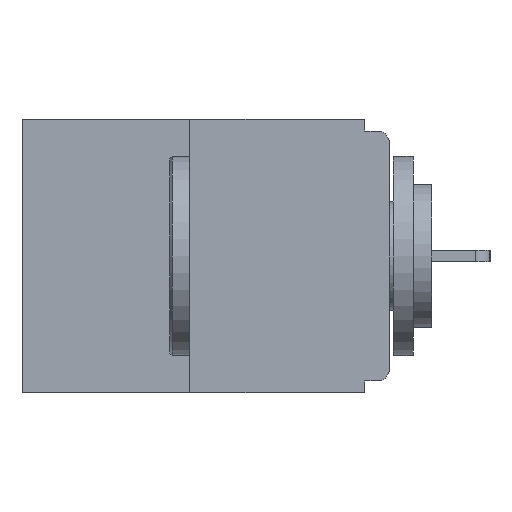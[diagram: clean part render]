
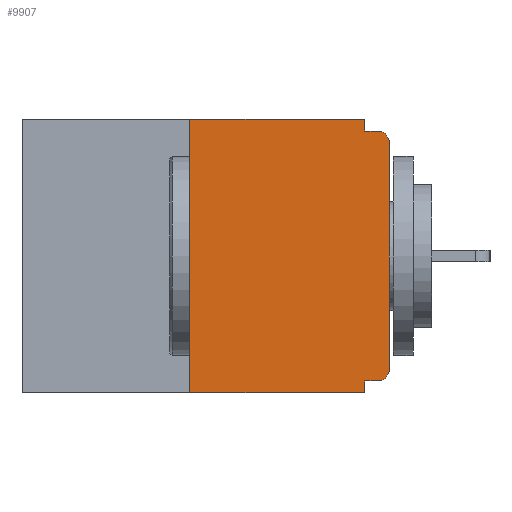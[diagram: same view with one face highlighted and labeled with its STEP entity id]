
A CAD part, left-side view. The second image highlights one B-rep face of the part: STEP entity #9907.
In plain terms, the highlighted planar face has unit normal (-1, 0, 0).
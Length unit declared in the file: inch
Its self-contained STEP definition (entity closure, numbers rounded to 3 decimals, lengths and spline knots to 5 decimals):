
#14 = CIRCLE ( 'NONE', #12090, 0.015 ) ;
#15 = VECTOR ( 'NONE', #4127, 39.37008 ) ;
#168 = VERTEX_POINT ( 'NONE', #7104 ) ;
#315 = CARTESIAN_POINT ( 'NONE',  ( 0., 0.031, -0.343 ) ) ;
#317 = VECTOR ( 'NONE', #24009, 39.37008 ) ;
#413 = CARTESIAN_POINT ( 'NONE',  ( 0., 0., -0.015 ) ) ;
#1266 = VERTEX_POINT ( 'NONE', #2147 ) ;
#1448 = ORIENTED_EDGE ( 'NONE', *, *, #12401, .F. ) ;
#2147 = CARTESIAN_POINT ( 'NONE',  ( 0., 0.031, -0.015 ) ) ;
#2425 = DIRECTION ( 'NONE',  ( 0., 0., -1. ) ) ;
#2603 = DIRECTION ( 'NONE',  ( 0., -1., 0. ) ) ;
#2755 = ORIENTED_EDGE ( 'NONE', *, *, #16962, .F. ) ;
#2942 = VERTEX_POINT ( 'NONE', #4803 ) ;
#3074 = EDGE_CURVE ( 'NONE', #17385, #5386, #14, .T. ) ;
#3148 = LINE ( 'NONE', #9006, #18382 ) ;
#3229 = AXIS2_PLACEMENT_3D ( 'NONE', #9556, #23301, #11506 ) ;
#4127 = DIRECTION ( 'NONE',  ( 0., -1., 0. ) ) ;
#4778 = VECTOR ( 'NONE', #25090, 39.37008 ) ;
#4803 = CARTESIAN_POINT ( 'NONE',  ( 0., 0.031, -0.328 ) ) ;
#5386 = VERTEX_POINT ( 'NONE', #9613 ) ;
#5591 = EDGE_LOOP ( 'NONE', ( #2755, #8173, #11188, #17680, #1448, #23832, #8790, #19927, #10609, #21147 ) ) ;
#5825 = EDGE_CURVE ( 'NONE', #1266, #168, #15173, .T. ) ;
#6660 = CARTESIAN_POINT ( 'NONE',  ( 0., 0.25, 0. ) ) ;
#7104 = CARTESIAN_POINT ( 'NONE',  ( 0., 0.015, -0.015 ) ) ;
#7207 = LINE ( 'NONE', #8399, #22310 ) ;
#8173 = ORIENTED_EDGE ( 'NONE', *, *, #24407, .F. ) ;
#8399 = CARTESIAN_POINT ( 'NONE',  ( 0., 0.46, -0.343 ) ) ;
#8790 = ORIENTED_EDGE ( 'NONE', *, *, #19071, .T. ) ;
#8882 = VERTEX_POINT ( 'NONE', #12332 ) ;
#9006 = CARTESIAN_POINT ( 'NONE',  ( 0., 0., 0. ) ) ;
#9134 = VECTOR ( 'NONE', #16734, 39.37008 ) ;
#9327 = CARTESIAN_POINT ( 'NONE',  ( 0., 0.015, -0.328 ) ) ;
#9354 = VERTEX_POINT ( 'NONE', #23588 ) ;
#9471 = DIRECTION ( 'NONE',  ( -1., 0., 0. ) ) ;
#9492 = CARTESIAN_POINT ( 'NONE',  ( 0., 0.031, 0. ) ) ;
#9556 = CARTESIAN_POINT ( 'NONE',  ( 0., 0.46, 0. ) ) ;
#9613 = CARTESIAN_POINT ( 'NONE',  ( 0., 0., -0.313 ) ) ;
#9907 = ADVANCED_FACE ( 'NONE', ( #16258 ), #17359, .F. ) ;
#10040 = CARTESIAN_POINT ( 'NONE',  ( 0., 0.46, 0. ) ) ;
#10048 = LINE ( 'NONE', #17209, #4778 ) ;
#10317 = LINE ( 'NONE', #315, #15488 ) ;
#10609 = ORIENTED_EDGE ( 'NONE', *, *, #5825, .F. ) ;
#10953 = DIRECTION ( 'NONE',  ( 0., 0., 1. ) ) ;
#11188 = ORIENTED_EDGE ( 'NONE', *, *, #21877, .T. ) ;
#11506 = DIRECTION ( 'NONE',  ( 0., 0., -1. ) ) ;
#12090 = AXIS2_PLACEMENT_3D ( 'NONE', #23966, #23925, #24396 ) ;
#12209 = CARTESIAN_POINT ( 'NONE',  ( 0., 0.25, 0. ) ) ;
#12332 = CARTESIAN_POINT ( 'NONE',  ( 0., 0.031, -0.343 ) ) ;
#12401 = EDGE_CURVE ( 'NONE', #17385, #2942, #24187, .T. ) ;
#12864 = VERTEX_POINT ( 'NONE', #24212 ) ;
#13393 = CIRCLE ( 'NONE', #21810, 0.015 ) ;
#14548 = VECTOR ( 'NONE', #2603, 39.37008 ) ;
#14709 = CARTESIAN_POINT ( 'NONE',  ( 0., 0., -0.328 ) ) ;
#15173 = LINE ( 'NONE', #413, #14548 ) ;
#15488 = VECTOR ( 'NONE', #2425, 39.37008 ) ;
#15620 = LINE ( 'NONE', #12209, #317 ) ;
#16258 = FACE_OUTER_BOUND ( 'NONE', #5591, .T. ) ;
#16734 = DIRECTION ( 'NONE',  ( 0., 1., 0. ) ) ;
#16753 = VERTEX_POINT ( 'NONE', #6660 ) ;
#16962 = EDGE_CURVE ( 'NONE', #16753, #17451, #21294, .T. ) ;
#17209 = CARTESIAN_POINT ( 'NONE',  ( 0., 0.031, 0. ) ) ;
#17359 = PLANE ( 'NONE',  #3229 ) ;
#17385 = VERTEX_POINT ( 'NONE', #9327 ) ;
#17451 = VERTEX_POINT ( 'NONE', #9492 ) ;
#17680 = ORIENTED_EDGE ( 'NONE', *, *, #20568, .F. ) ;
#18382 = VECTOR ( 'NONE', #10953, 39.37008 ) ;
#19071 = EDGE_CURVE ( 'NONE', #5386, #12864, #3148, .T. ) ;
#19230 = EDGE_CURVE ( 'NONE', #17451, #1266, #10048, .T. ) ;
#19927 = ORIENTED_EDGE ( 'NONE', *, *, #24735, .T. ) ;
#20392 = DIRECTION ( 'NONE',  ( 0., -1., 0. ) ) ;
#20568 = EDGE_CURVE ( 'NONE', #2942, #8882, #10317, .T. ) ;
#21147 = ORIENTED_EDGE ( 'NONE', *, *, #19230, .F. ) ;
#21294 = LINE ( 'NONE', #10040, #15 ) ;
#21314 = CARTESIAN_POINT ( 'NONE',  ( 0., 0.015, -0.03 ) ) ;
#21810 = AXIS2_PLACEMENT_3D ( 'NONE', #21314, #9471, #23222 ) ;
#21877 = EDGE_CURVE ( 'NONE', #9354, #8882, #7207, .T. ) ;
#22310 = VECTOR ( 'NONE', #20392, 39.37008 ) ;
#23222 = DIRECTION ( 'NONE',  ( 0., 0., -1. ) ) ;
#23301 = DIRECTION ( 'NONE',  ( 1., 0., 0. ) ) ;
#23588 = CARTESIAN_POINT ( 'NONE',  ( 0., 0.25, -0.343 ) ) ;
#23832 = ORIENTED_EDGE ( 'NONE', *, *, #3074, .T. ) ;
#23925 = DIRECTION ( 'NONE',  ( -1., 0., 0. ) ) ;
#23966 = CARTESIAN_POINT ( 'NONE',  ( 0., 0.015, -0.313 ) ) ;
#24009 = DIRECTION ( 'NONE',  ( 0., 0., 1. ) ) ;
#24187 = LINE ( 'NONE', #14709, #9134 ) ;
#24212 = CARTESIAN_POINT ( 'NONE',  ( 0., 0., -0.03 ) ) ;
#24396 = DIRECTION ( 'NONE',  ( 0., 0., -1. ) ) ;
#24407 = EDGE_CURVE ( 'NONE', #9354, #16753, #15620, .T. ) ;
#24735 = EDGE_CURVE ( 'NONE', #12864, #168, #13393, .T. ) ;
#25090 = DIRECTION ( 'NONE',  ( 0., 0., -1. ) ) ;
